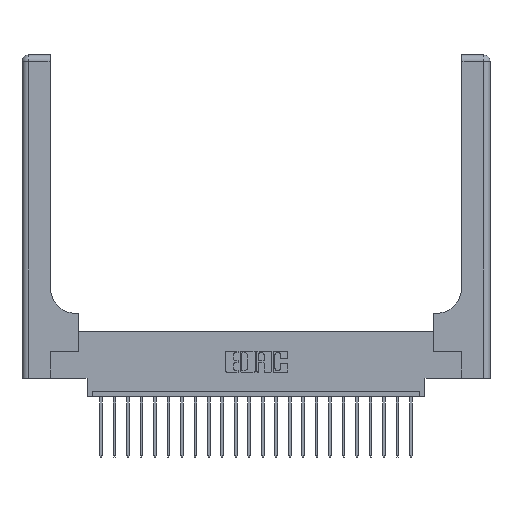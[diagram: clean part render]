
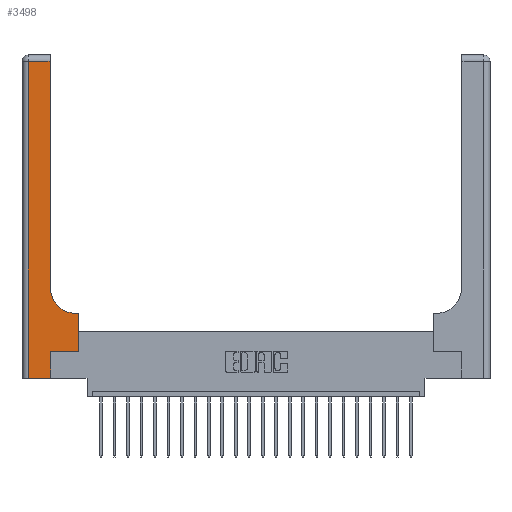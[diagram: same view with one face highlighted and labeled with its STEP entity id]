
A CAD part, top view. The second image highlights one B-rep face of the part: STEP entity #3498.
In plain terms, the highlighted planar face has unit normal (0, 0, 1).
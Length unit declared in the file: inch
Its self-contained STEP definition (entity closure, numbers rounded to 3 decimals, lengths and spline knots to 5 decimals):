
#175 = EDGE_CURVE ( 'NONE', #13255, #22019, #7687, .T. ) ;
#240 = EDGE_LOOP ( 'NONE', ( #19752, #3448, #15366, #10280, #12839, #4057, #6607, #11729, #20795 ) ) ;
#289 = DIRECTION ( 'NONE',  ( 0., 1., 0. ) ) ;
#1275 = VERTEX_POINT ( 'NONE', #4973 ) ;
#1729 = EDGE_CURVE ( 'NONE', #22019, #3183, #12282, .T. ) ;
#2370 = CARTESIAN_POINT ( 'NONE',  ( 0.26, 0.85, 0.37 ) ) ;
#2681 = EDGE_CURVE ( 'NONE', #17745, #9127, #6504, .T. ) ;
#2721 = DIRECTION ( 'NONE',  ( -1., 0., 0. ) ) ;
#3183 = VERTEX_POINT ( 'NONE', #7056 ) ;
#3448 = ORIENTED_EDGE ( 'NONE', *, *, #175, .T. ) ;
#3498 = ADVANCED_FACE ( 'NONE', ( #6331 ), #22218, .F. ) ;
#4057 = ORIENTED_EDGE ( 'NONE', *, *, #16932, .T. ) ;
#4072 = DIRECTION ( 'NONE',  ( -1., 0., 0. ) ) ;
#4097 = VECTOR ( 'NONE', #289, 39.37008 ) ;
#4363 = DIRECTION ( 'NONE',  ( 0., 1., 0. ) ) ;
#4879 = DIRECTION ( 'NONE',  ( 0., 1., 0. ) ) ;
#4973 = CARTESIAN_POINT ( 'NONE',  ( 0.528, 0.25, 0.37 ) ) ;
#5418 = CARTESIAN_POINT ( 'NONE',  ( 0.51, 0.85, 0.37 ) ) ;
#5944 = EDGE_CURVE ( 'NONE', #6428, #7049, #11488, .T. ) ;
#6331 = FACE_OUTER_BOUND ( 'NONE', #240, .T. ) ;
#6428 = VERTEX_POINT ( 'NONE', #9715 ) ;
#6504 = LINE ( 'NONE', #15491, #17623 ) ;
#6607 = ORIENTED_EDGE ( 'NONE', *, *, #12254, .T. ) ;
#7049 = VERTEX_POINT ( 'NONE', #17835 ) ;
#7056 = CARTESIAN_POINT ( 'NONE',  ( 0.06, 0., 0.37 ) ) ;
#7171 = VECTOR ( 'NONE', #4072, 39.37008 ) ;
#7687 = LINE ( 'NONE', #9549, #7171 ) ;
#8807 = EDGE_CURVE ( 'NONE', #3183, #6428, #19553, .T. ) ;
#9127 = VERTEX_POINT ( 'NONE', #14204 ) ;
#9549 = CARTESIAN_POINT ( 'NONE',  ( 0., 2.94, 0.37 ) ) ;
#9715 = CARTESIAN_POINT ( 'NONE',  ( 0.265, 0., 0.37 ) ) ;
#9746 = CARTESIAN_POINT ( 'NONE',  ( 0.06, 3., 0.37 ) ) ;
#10230 = LINE ( 'NONE', #21221, #16863 ) ;
#10280 = ORIENTED_EDGE ( 'NONE', *, *, #8807, .T. ) ;
#10596 = CARTESIAN_POINT ( 'NONE',  ( 0.26, 3., 0.37 ) ) ;
#10669 = CARTESIAN_POINT ( 'NONE',  ( 0., 0., 0.37 ) ) ;
#11230 = CIRCLE ( 'NONE', #14576, 0.25 ) ;
#11488 = LINE ( 'NONE', #14881, #14354 ) ;
#11527 = CARTESIAN_POINT ( 'NONE',  ( 0.06, 2.94, 0.37 ) ) ;
#11712 = EDGE_CURVE ( 'NONE', #13172, #13255, #19595, .T. ) ;
#11729 = ORIENTED_EDGE ( 'NONE', *, *, #2681, .T. ) ;
#12254 = EDGE_CURVE ( 'NONE', #1275, #17745, #19920, .T. ) ;
#12282 = LINE ( 'NONE', #9746, #18538 ) ;
#12284 = VECTOR ( 'NONE', #4879, 39.37008 ) ;
#12839 = ORIENTED_EDGE ( 'NONE', *, *, #5944, .T. ) ;
#13172 = VERTEX_POINT ( 'NONE', #2370 ) ;
#13255 = VERTEX_POINT ( 'NONE', #18808 ) ;
#13680 = DIRECTION ( 'NONE',  ( 0., 0., -1. ) ) ;
#14185 = DIRECTION ( 'NONE',  ( 1., 0., 0. ) ) ;
#14198 = DIRECTION ( 'NONE',  ( 1., 0., 0. ) ) ;
#14204 = CARTESIAN_POINT ( 'NONE',  ( 0.51, 0.6, 0.37 ) ) ;
#14354 = VECTOR ( 'NONE', #4363, 39.37008 ) ;
#14576 = AXIS2_PLACEMENT_3D ( 'NONE', #5418, #20036, #14185 ) ;
#14881 = CARTESIAN_POINT ( 'NONE',  ( 0.265, 0., 0.37 ) ) ;
#15063 = CARTESIAN_POINT ( 'NONE',  ( 0.528, 0.25, 0.37 ) ) ;
#15366 = ORIENTED_EDGE ( 'NONE', *, *, #1729, .T. ) ;
#15491 = CARTESIAN_POINT ( 'NONE',  ( 0.26, 0.6, 0.37 ) ) ;
#15752 = EDGE_CURVE ( 'NONE', #9127, #13172, #11230, .T. ) ;
#15894 = DIRECTION ( 'NONE',  ( 0., -1., 0. ) ) ;
#16400 = DIRECTION ( 'NONE',  ( 1., 0., 0. ) ) ;
#16863 = VECTOR ( 'NONE', #14198, 39.37008 ) ;
#16932 = EDGE_CURVE ( 'NONE', #7049, #1275, #10230, .T. ) ;
#17623 = VECTOR ( 'NONE', #19133, 39.37008 ) ;
#17745 = VERTEX_POINT ( 'NONE', #20937 ) ;
#17835 = CARTESIAN_POINT ( 'NONE',  ( 0.265, 0.25, 0.37 ) ) ;
#18538 = VECTOR ( 'NONE', #15894, 39.37008 ) ;
#18722 = CARTESIAN_POINT ( 'NONE',  ( 0., 3., 0.37 ) ) ;
#18808 = CARTESIAN_POINT ( 'NONE',  ( 0.26, 2.94, 0.37 ) ) ;
#19133 = DIRECTION ( 'NONE',  ( -1., 0., 0. ) ) ;
#19553 = LINE ( 'NONE', #10669, #20090 ) ;
#19595 = LINE ( 'NONE', #10596, #12284 ) ;
#19752 = ORIENTED_EDGE ( 'NONE', *, *, #11712, .T. ) ;
#19920 = LINE ( 'NONE', #15063, #4097 ) ;
#20036 = DIRECTION ( 'NONE',  ( 0., 0., -1. ) ) ;
#20090 = VECTOR ( 'NONE', #16400, 39.37008 ) ;
#20795 = ORIENTED_EDGE ( 'NONE', *, *, #15752, .T. ) ;
#20937 = CARTESIAN_POINT ( 'NONE',  ( 0.528, 0.6, 0.37 ) ) ;
#21221 = CARTESIAN_POINT ( 'NONE',  ( 0.265, 0.25, 0.37 ) ) ;
#22019 = VERTEX_POINT ( 'NONE', #11527 ) ;
#22162 = AXIS2_PLACEMENT_3D ( 'NONE', #18722, #13680, #2721 ) ;
#22218 = PLANE ( 'NONE',  #22162 ) ;
